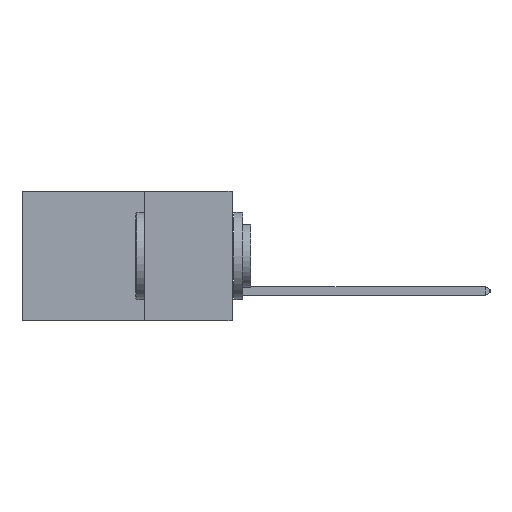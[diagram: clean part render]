
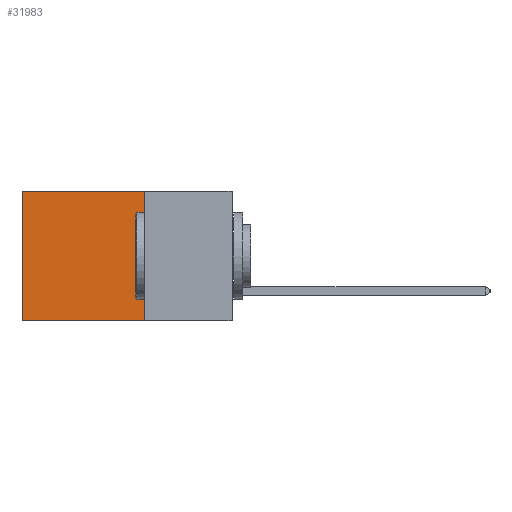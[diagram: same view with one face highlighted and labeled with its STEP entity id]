
A CAD part, left-side view. The second image highlights one B-rep face of the part: STEP entity #31983.
In plain terms, the highlighted planar face has unit normal (-1, 0, 0).
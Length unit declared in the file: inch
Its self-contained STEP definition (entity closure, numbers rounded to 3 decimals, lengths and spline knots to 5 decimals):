
#1953 = PLANE ( 'NONE',  #10940 ) ;
#2447 = VECTOR ( 'NONE', #17553, 39.37008 ) ;
#3030 = DIRECTION ( 'NONE',  ( 0., 1., 0. ) ) ;
#5022 = DIRECTION ( 'NONE',  ( 0., 0., -1. ) ) ;
#5764 = DIRECTION ( 'NONE',  ( 0., 1., 0. ) ) ;
#8797 = VERTEX_POINT ( 'NONE', #37219 ) ;
#10591 = VECTOR ( 'NONE', #11485, 39.37008 ) ;
#10940 = AXIS2_PLACEMENT_3D ( 'NONE', #17222, #23392, #5022 ) ;
#11116 = ORIENTED_EDGE ( 'NONE', *, *, #39190, .T. ) ;
#11125 = EDGE_CURVE ( 'NONE', #13278, #12617, #20610, .T. ) ;
#11430 = CARTESIAN_POINT ( 'NONE',  ( 0.2875, 0.6, -0.37 ) ) ;
#11485 = DIRECTION ( 'NONE',  ( 0., 0., -1. ) ) ;
#12617 = VERTEX_POINT ( 'NONE', #22346 ) ;
#13278 = VERTEX_POINT ( 'NONE', #22972 ) ;
#17222 = CARTESIAN_POINT ( 'NONE',  ( 0.2875, 0.25, 0. ) ) ;
#17445 = ORIENTED_EDGE ( 'NONE', *, *, #34535, .F. ) ;
#17553 = DIRECTION ( 'NONE',  ( 0., 0., -1. ) ) ;
#17809 = LINE ( 'NONE', #38773, #10591 ) ;
#20011 = ORIENTED_EDGE ( 'NONE', *, *, #11125, .T. ) ;
#20610 = LINE ( 'NONE', #24459, #28726 ) ;
#22346 = CARTESIAN_POINT ( 'NONE',  ( 0.2875, 0.6, 0. ) ) ;
#22972 = CARTESIAN_POINT ( 'NONE',  ( 0.2875, 0.25, 0. ) ) ;
#23392 = DIRECTION ( 'NONE',  ( 1., 0., 0. ) ) ;
#24459 = CARTESIAN_POINT ( 'NONE',  ( 0.2875, 0.25, 0. ) ) ;
#24980 = LINE ( 'NONE', #32695, #2447 ) ;
#27209 = CARTESIAN_POINT ( 'NONE',  ( 0.2875, 0.25, -0.37 ) ) ;
#28726 = VECTOR ( 'NONE', #3030, 39.37008 ) ;
#30041 = LINE ( 'NONE', #27209, #37114 ) ;
#31227 = FACE_OUTER_BOUND ( 'NONE', #32212, .T. ) ;
#31983 = ADVANCED_FACE ( 'NONE', ( #31227 ), #1953, .F. ) ;
#32078 = VERTEX_POINT ( 'NONE', #11430 ) ;
#32212 = EDGE_LOOP ( 'NONE', ( #11116, #17445, #35850, #20011 ) ) ;
#32695 = CARTESIAN_POINT ( 'NONE',  ( 0.2875, 0.6, 0. ) ) ;
#33223 = EDGE_CURVE ( 'NONE', #13278, #8797, #17809, .T. ) ;
#34535 = EDGE_CURVE ( 'NONE', #8797, #32078, #30041, .T. ) ;
#35850 = ORIENTED_EDGE ( 'NONE', *, *, #33223, .F. ) ;
#37114 = VECTOR ( 'NONE', #5764, 39.37008 ) ;
#37219 = CARTESIAN_POINT ( 'NONE',  ( 0.2875, 0.25, -0.37 ) ) ;
#38773 = CARTESIAN_POINT ( 'NONE',  ( 0.2875, 0.25, 0. ) ) ;
#39190 = EDGE_CURVE ( 'NONE', #12617, #32078, #24980, .T. ) ;
